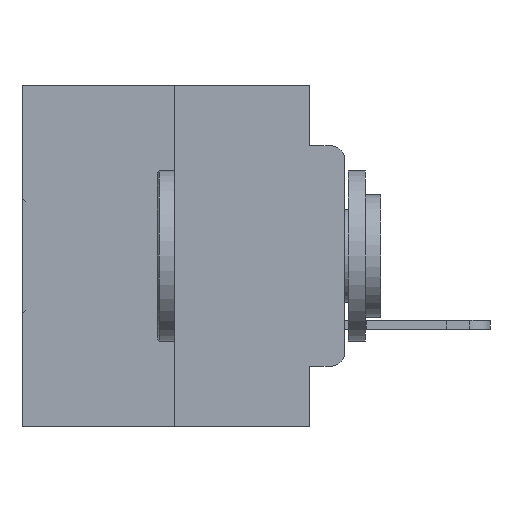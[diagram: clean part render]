
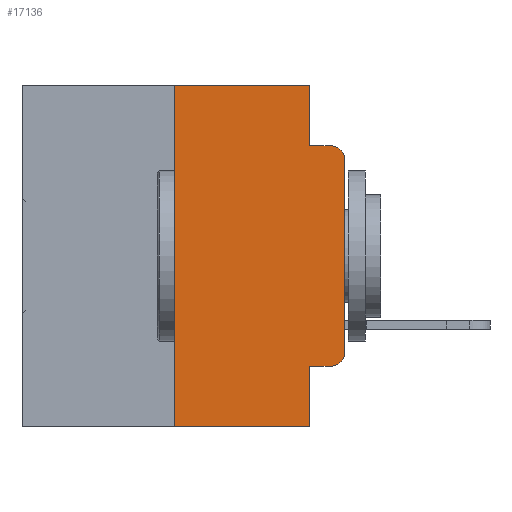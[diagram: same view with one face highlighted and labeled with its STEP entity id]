
A CAD part, left-side view. The second image highlights one B-rep face of the part: STEP entity #17136.
In plain terms, the highlighted planar face has unit normal (-1, 0, 0).
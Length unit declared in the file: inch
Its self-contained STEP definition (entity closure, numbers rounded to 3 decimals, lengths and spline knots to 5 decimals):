
#817 = VERTEX_POINT ( 'NONE', #4801 ) ;
#957 = VERTEX_POINT ( 'NONE', #6875 ) ;
#2074 = AXIS2_PLACEMENT_3D ( 'NONE', #26088, #25884, #25911 ) ;
#2741 = CARTESIAN_POINT ( 'NONE',  ( 0., 0., -0.3915 ) ) ;
#2910 = CIRCLE ( 'NONE', #2074, 0.02 ) ;
#3070 = DIRECTION ( 'NONE',  ( 0., -1., 0. ) ) ;
#3298 = CARTESIAN_POINT ( 'NONE',  ( 0., 0.051, -0.0885 ) ) ;
#4121 = ORIENTED_EDGE ( 'NONE', *, *, #10063, .T. ) ;
#4365 = CARTESIAN_POINT ( 'NONE',  ( 0., 0.051, -0.4115 ) ) ;
#4801 = CARTESIAN_POINT ( 'NONE',  ( 0., 0.051, -0.5 ) ) ;
#4922 = LINE ( 'NONE', #10013, #8530 ) ;
#5058 = ORIENTED_EDGE ( 'NONE', *, *, #9769, .F. ) ;
#5203 = CARTESIAN_POINT ( 'NONE',  ( 0., 0.051, -0.4115 ) ) ;
#5473 = ORIENTED_EDGE ( 'NONE', *, *, #9918, .F. ) ;
#5690 = VERTEX_POINT ( 'NONE', #5203 ) ;
#5839 = LINE ( 'NONE', #20026, #30818 ) ;
#6281 = CARTESIAN_POINT ( 'NONE',  ( 0., 0.02, -0.0885 ) ) ;
#6493 = DIRECTION ( 'NONE',  ( 0., 0., -1. ) ) ;
#6525 = VERTEX_POINT ( 'NONE', #3298 ) ;
#6727 = LINE ( 'NONE', #15917, #19240 ) ;
#6875 = CARTESIAN_POINT ( 'NONE',  ( 0., 0.051, 0. ) ) ;
#7961 = CARTESIAN_POINT ( 'NONE',  ( 0., 0.051, 0. ) ) ;
#8232 = VECTOR ( 'NONE', #24707, 39.37008 ) ;
#8530 = VECTOR ( 'NONE', #15048, 39.37008 ) ;
#8834 = DIRECTION ( 'NONE',  ( 0., 0., 1. ) ) ;
#8997 = CARTESIAN_POINT ( 'NONE',  ( 0., 0.25, 0. ) ) ;
#9040 = LINE ( 'NONE', #30380, #8232 ) ;
#9577 = EDGE_CURVE ( 'NONE', #26126, #29347, #31159, .T. ) ;
#9629 = EDGE_CURVE ( 'NONE', #29347, #11204, #2910, .T. ) ;
#9682 = EDGE_CURVE ( 'NONE', #6525, #11204, #9040, .T. ) ;
#9683 = ORIENTED_EDGE ( 'NONE', *, *, #9968, .T. ) ;
#9769 = EDGE_CURVE ( 'NONE', #957, #6525, #5839, .T. ) ;
#9918 = EDGE_CURVE ( 'NONE', #25229, #22493, #31137, .T. ) ;
#9957 = EDGE_CURVE ( 'NONE', #5690, #817, #12174, .T. ) ;
#9968 = EDGE_CURVE ( 'NONE', #5690, #21429, #29133, .T. ) ;
#10013 = CARTESIAN_POINT ( 'NONE',  ( 0., 0.473, -0.5 ) ) ;
#10063 = EDGE_CURVE ( 'NONE', #21429, #26126, #14901, .T. ) ;
#10136 = ORIENTED_EDGE ( 'NONE', *, *, #9682, .F. ) ;
#11204 = VERTEX_POINT ( 'NONE', #6281 ) ;
#11300 = ORIENTED_EDGE ( 'NONE', *, *, #9629, .T. ) ;
#11470 = PLANE ( 'NONE',  #18834 ) ;
#12174 = LINE ( 'NONE', #7961, #29787 ) ;
#14602 = ORIENTED_EDGE ( 'NONE', *, *, #15847, .T. ) ;
#14901 = CIRCLE ( 'NONE', #28522, 0.02 ) ;
#15048 = DIRECTION ( 'NONE',  ( 0., -1., 0. ) ) ;
#15847 = EDGE_CURVE ( 'NONE', #25229, #817, #4922, .T. ) ;
#15917 = CARTESIAN_POINT ( 'NONE',  ( 0., 0.473, 0. ) ) ;
#15926 = CARTESIAN_POINT ( 'NONE',  ( 0., 0.25, -0.5 ) ) ;
#16465 = DIRECTION ( 'NONE',  ( 0., 0., -1. ) ) ;
#16730 = ORIENTED_EDGE ( 'NONE', *, *, #9577, .T. ) ;
#17136 = ADVANCED_FACE ( 'NONE', ( #18715 ), #11470, .F. ) ;
#18612 = CARTESIAN_POINT ( 'NONE',  ( 0., 0., -0.1085 ) ) ;
#18715 = FACE_OUTER_BOUND ( 'NONE', #31236, .T. ) ;
#18834 = AXIS2_PLACEMENT_3D ( 'NONE', #23731, #30581, #16465 ) ;
#19240 = VECTOR ( 'NONE', #30126, 39.37008 ) ;
#19528 = VECTOR ( 'NONE', #8834, 39.37008 ) ;
#19932 = DIRECTION ( 'NONE',  ( 0., 0., -1. ) ) ;
#20026 = CARTESIAN_POINT ( 'NONE',  ( 0., 0.051, 0. ) ) ;
#21429 = VERTEX_POINT ( 'NONE', #25746 ) ;
#21537 = ORIENTED_EDGE ( 'NONE', *, *, #23408, .F. ) ;
#22177 = CARTESIAN_POINT ( 'NONE',  ( 0., 0.25, 0. ) ) ;
#22493 = VERTEX_POINT ( 'NONE', #22177 ) ;
#23408 = EDGE_CURVE ( 'NONE', #22493, #957, #6727, .T. ) ;
#23731 = CARTESIAN_POINT ( 'NONE',  ( 0., 0.473, 0. ) ) ;
#23808 = VECTOR ( 'NONE', #3070, 39.37008 ) ;
#24707 = DIRECTION ( 'NONE',  ( 0., -1., 0. ) ) ;
#25229 = VERTEX_POINT ( 'NONE', #15926 ) ;
#25547 = ORIENTED_EDGE ( 'NONE', *, *, #9957, .F. ) ;
#25746 = CARTESIAN_POINT ( 'NONE',  ( 0., 0.02, -0.4115 ) ) ;
#25884 = DIRECTION ( 'NONE',  ( -1., 0., 0. ) ) ;
#25911 = DIRECTION ( 'NONE',  ( 0., 0., -1. ) ) ;
#26088 = CARTESIAN_POINT ( 'NONE',  ( 0., 0.02, -0.1085 ) ) ;
#26126 = VERTEX_POINT ( 'NONE', #2741 ) ;
#28522 = AXIS2_PLACEMENT_3D ( 'NONE', #31192, #31151, #31123 ) ;
#29133 = LINE ( 'NONE', #4365, #23808 ) ;
#29347 = VERTEX_POINT ( 'NONE', #18612 ) ;
#29787 = VECTOR ( 'NONE', #6493, 39.37008 ) ;
#30126 = DIRECTION ( 'NONE',  ( 0., -1., 0. ) ) ;
#30232 = CARTESIAN_POINT ( 'NONE',  ( 0., 0., 0. ) ) ;
#30380 = CARTESIAN_POINT ( 'NONE',  ( 0., 0.051, -0.0885 ) ) ;
#30483 = VECTOR ( 'NONE', #30601, 39.37008 ) ;
#30581 = DIRECTION ( 'NONE',  ( 1., 0., 0. ) ) ;
#30601 = DIRECTION ( 'NONE',  ( 0., 0., 1. ) ) ;
#30818 = VECTOR ( 'NONE', #19932, 39.37008 ) ;
#31123 = DIRECTION ( 'NONE',  ( 0., 0., -1. ) ) ;
#31137 = LINE ( 'NONE', #8997, #19528 ) ;
#31151 = DIRECTION ( 'NONE',  ( -1., 0., 0. ) ) ;
#31159 = LINE ( 'NONE', #30232, #30483 ) ;
#31192 = CARTESIAN_POINT ( 'NONE',  ( 0., 0.02, -0.3915 ) ) ;
#31236 = EDGE_LOOP ( 'NONE', ( #16730, #11300, #10136, #5058, #21537, #5473, #14602, #25547, #9683, #4121 ) ) ;
